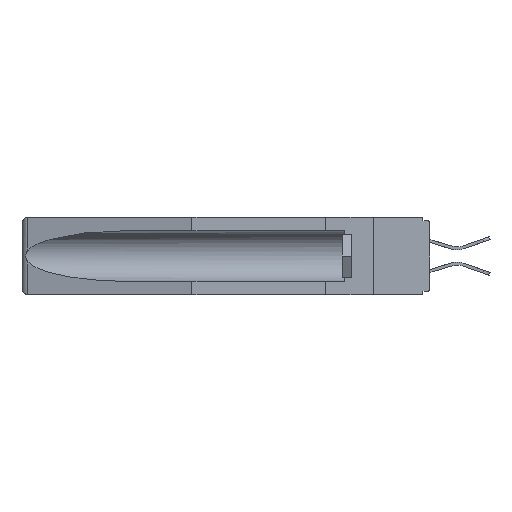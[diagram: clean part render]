
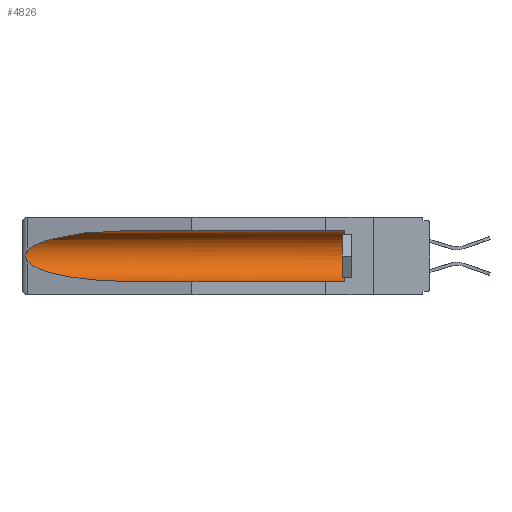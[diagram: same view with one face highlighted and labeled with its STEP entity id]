
A CAD part, left-side view. The second image highlights one B-rep face of the part: STEP entity #4826.
In plain terms, the highlighted cylindrical face has radius 2.857 mm (diameter 5.715 mm), a partial arc.
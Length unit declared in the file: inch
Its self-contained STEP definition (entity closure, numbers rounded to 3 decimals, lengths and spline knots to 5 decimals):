
#150 = CARTESIAN_POINT ( 'NONE',  ( 0.2675, 1.53308, -0.16763 ) ) ;
#827 = CARTESIAN_POINT ( 'NONE',  ( 0.26537, 1.52718, -0.19328 ) ) ;
#858 = ORIENTED_EDGE ( 'NONE', *, *, #19139, .T. ) ;
#948 = CARTESIAN_POINT ( 'NONE',  ( 0.155, -0.30754, -0.284 ) ) ;
#1108 = AXIS2_PLACEMENT_3D ( 'NONE', #22662, #15032, #12325 ) ;
#1174 = DIRECTION ( 'NONE',  ( 0., 1., 0. ) ) ;
#3330 = CARTESIAN_POINT ( 'NONE',  ( 0.21114, 1.30732, -0.284 ) ) ;
#3358 = LINE ( 'NONE', #948, #13087 ) ;
#3434 = CARTESIAN_POINT ( 'NONE',  ( 0.155, 1.07973, -0.284 ) ) ;
#4219 = FACE_OUTER_BOUND ( 'NONE', #30974, .T. ) ;
#4826 = ADVANCED_FACE ( 'NONE', ( #4219 ), #24445, .F. ) ;
#5039 = CARTESIAN_POINT ( 'NONE',  ( 0.26537, 1.52718, -0.14972 ) ) ;
#5150 = CARTESIAN_POINT ( 'NONE',  ( 0.26537, 1.52718, -0.19328 ) ) ;
#5257 = CARTESIAN_POINT ( 'NONE',  ( 0.26654, 1.53092, -0.15636 ) ) ;
#6400 = CARTESIAN_POINT ( 'NONE',  ( 0.155, 0.126, -0.059 ) ) ;
#7804 = LINE ( 'NONE', #23689, #16380 ) ;
#7969 = CARTESIAN_POINT ( 'NONE',  ( 0.26655, 1.53094, -0.18657 ) ) ;
#10142 =( BOUNDED_CURVE ( )  B_SPLINE_CURVE ( 3, ( #827, #10819, #3330, #3434 ),
 .UNSPECIFIED., .F., .F. ) 
 B_SPLINE_CURVE_WITH_KNOTS ( ( 4, 4 ),
 ( 0.1948, 1.5708 ),
 .UNSPECIFIED. ) 
 CURVE ( )  GEOMETRIC_REPRESENTATION_ITEM ( )  RATIONAL_B_SPLINE_CURVE ( ( 1., 0.848, 0.848, 1. ) ) 
 REPRESENTATION_ITEM ( '' )  );
#10780 = CARTESIAN_POINT ( 'NONE',  ( 0.155, 1.07973, -0.059 ) ) ;
#10819 = CARTESIAN_POINT ( 'NONE',  ( 0.25451, 1.48313, -0.24835 ) ) ;
#12325 = DIRECTION ( 'NONE',  ( 0., 0., 1. ) ) ;
#13087 = VECTOR ( 'NONE', #1174, 39.37008 ) ;
#13183 = CARTESIAN_POINT ( 'NONE',  ( 0.26537, 1.52718, -0.19328 ) ) ;
#13687 = DIRECTION ( 'NONE',  ( 0., 1., 0. ) ) ;
#14860 = VERTEX_POINT ( 'NONE', #13183 ) ;
#14909 =( BOUNDED_CURVE ( )  B_SPLINE_CURVE ( 3, ( #27693, #20283, #30400, #28007 ),
 .UNSPECIFIED., .F., .F. ) 
 B_SPLINE_CURVE_WITH_KNOTS ( ( 4, 4 ),
 ( 4.71239, 6.08839 ),
 .UNSPECIFIED. ) 
 CURVE ( )  GEOMETRIC_REPRESENTATION_ITEM ( )  RATIONAL_B_SPLINE_CURVE ( ( 1., 0.848, 0.848, 1. ) ) 
 REPRESENTATION_ITEM ( '' )  );
#15032 = DIRECTION ( 'NONE',  ( 0., -1., 0. ) ) ;
#15159 = CARTESIAN_POINT ( 'NONE',  ( 0.2673, 1.5327, -0.16383 ) ) ;
#16380 = VECTOR ( 'NONE', #13687, 39.37008 ) ;
#17244 = VERTEX_POINT ( 'NONE', #17625 ) ;
#17316 = VERTEX_POINT ( 'NONE', #30764 ) ;
#17451 = CARTESIAN_POINT ( 'NONE',  ( 0.26597, 1.52961, -0.15275 ) ) ;
#17557 = CARTESIAN_POINT ( 'NONE',  ( 0.2675, 1.53308, -0.17534 ) ) ;
#17625 = CARTESIAN_POINT ( 'NONE',  ( 0.26537, 1.52718, -0.14972 ) ) ;
#18731 = B_SPLINE_CURVE_WITH_KNOTS ( 'NONE', 3,
 ( #5039, #17451, #5257, #15159, #150, #17557, #27884, #7969, #24954, #5150 ),
 .UNSPECIFIED., .F., .F.,
 ( 4, 2, 2, 2, 4 ),
 ( 0., 0.00029, 0.00058, 0.00087, 0.00117 ),
 .UNSPECIFIED. ) ;
#18981 = VERTEX_POINT ( 'NONE', #27034 ) ;
#19139 = EDGE_CURVE ( 'NONE', #17244, #14860, #18731, .T. ) ;
#20283 = CARTESIAN_POINT ( 'NONE',  ( 0.21114, 1.30732, -0.059 ) ) ;
#20856 = ORIENTED_EDGE ( 'NONE', *, *, #23340, .T. ) ;
#20865 = ORIENTED_EDGE ( 'NONE', *, *, #28922, .T. ) ;
#21085 = DIRECTION ( 'NONE',  ( 0., 0., 1. ) ) ;
#22662 = CARTESIAN_POINT ( 'NONE',  ( 0.155, 0.126, -0.1715 ) ) ;
#23340 = EDGE_CURVE ( 'NONE', #25128, #17244, #14909, .T. ) ;
#23424 = EDGE_CURVE ( 'NONE', #14860, #18981, #10142, .T. ) ;
#23473 = CARTESIAN_POINT ( 'NONE',  ( 0.155, -0.30754, -0.1715 ) ) ;
#23581 = DIRECTION ( 'NONE',  ( 0., 1., 0. ) ) ;
#23689 = CARTESIAN_POINT ( 'NONE',  ( 0.155, -0.30754, -0.059 ) ) ;
#23699 = ORIENTED_EDGE ( 'NONE', *, *, #26822, .T. ) ;
#24445 = CYLINDRICAL_SURFACE ( 'NONE', #32012, 0.1125 ) ;
#24954 = CARTESIAN_POINT ( 'NONE',  ( 0.26597, 1.5296, -0.19026 ) ) ;
#25128 = VERTEX_POINT ( 'NONE', #10780 ) ;
#26594 = ORIENTED_EDGE ( 'NONE', *, *, #31805, .F. ) ;
#26822 = EDGE_CURVE ( 'NONE', #17316, #29007, #28217, .T. ) ;
#27034 = CARTESIAN_POINT ( 'NONE',  ( 0.155, 1.07973, -0.284 ) ) ;
#27693 = CARTESIAN_POINT ( 'NONE',  ( 0.155, 1.07973, -0.059 ) ) ;
#27884 = CARTESIAN_POINT ( 'NONE',  ( 0.2673, 1.53269, -0.17917 ) ) ;
#28007 = CARTESIAN_POINT ( 'NONE',  ( 0.26537, 1.52718, -0.14972 ) ) ;
#28217 = CIRCLE ( 'NONE', #1108, 0.1125 ) ;
#28922 = EDGE_CURVE ( 'NONE', #29007, #25128, #7804, .T. ) ;
#29007 = VERTEX_POINT ( 'NONE', #6400 ) ;
#29072 = ORIENTED_EDGE ( 'NONE', *, *, #23424, .T. ) ;
#30400 = CARTESIAN_POINT ( 'NONE',  ( 0.25451, 1.48313, -0.09465 ) ) ;
#30764 = CARTESIAN_POINT ( 'NONE',  ( 0.155, 0.126, -0.284 ) ) ;
#30974 = EDGE_LOOP ( 'NONE', ( #20856, #858, #29072, #26594, #23699, #20865 ) ) ;
#31805 = EDGE_CURVE ( 'NONE', #17316, #18981, #3358, .T. ) ;
#32012 = AXIS2_PLACEMENT_3D ( 'NONE', #23473, #23581, #21085 ) ;
